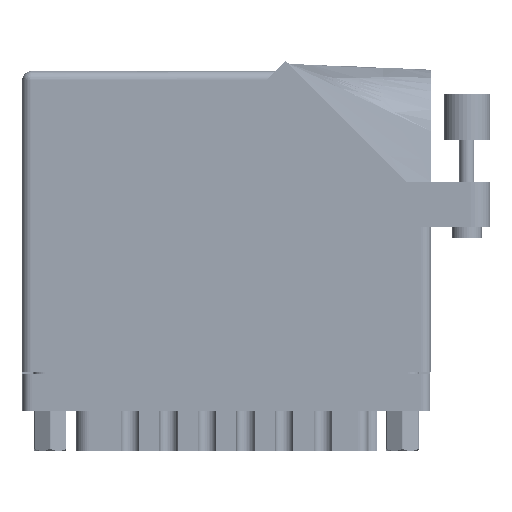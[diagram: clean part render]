
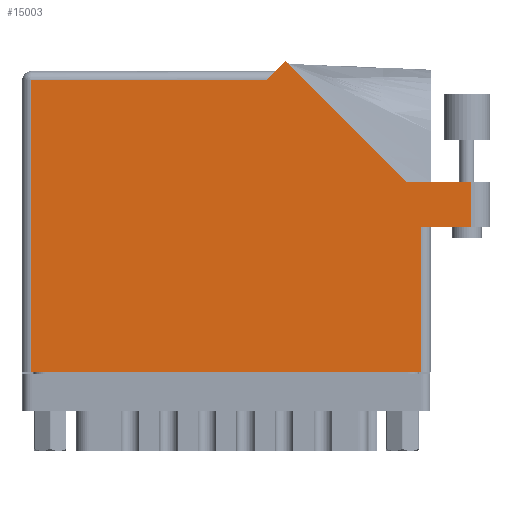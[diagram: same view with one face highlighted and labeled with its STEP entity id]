
A CAD part, front view. The second image highlights one B-rep face of the part: STEP entity #15003.
In plain terms, the highlighted face is planar.
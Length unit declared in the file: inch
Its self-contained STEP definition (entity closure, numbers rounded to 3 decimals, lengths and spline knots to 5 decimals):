
#31 = VECTOR ( 'NONE', #86775, 39.37008 ) ;
#2384 = ORIENTED_EDGE ( 'NONE', *, *, #24956, .T. ) ;
#2831 = ORIENTED_EDGE ( 'NONE', *, *, #23127, .T. ) ;
#3071 = VERTEX_POINT ( 'NONE', #104858 ) ;
#3099 = VECTOR ( 'NONE', #7529, 39.37008 ) ;
#4959 = CARTESIAN_POINT ( 'NONE',  ( 2.693, 0.98, 0. ) ) ;
#7529 = DIRECTION ( 'NONE',  ( 0., -1., 0. ) ) ;
#8479 = EDGE_CURVE ( 'NONE', #53730, #66438, #96730, .T. ) ;
#8989 = ORIENTED_EDGE ( 'NONE', *, *, #78465, .T. ) ;
#9529 = VERTEX_POINT ( 'NONE', #45288 ) ;
#11699 = DIRECTION ( 'NONE',  ( -1., 0., 0. ) ) ;
#15003 = ADVANCED_FACE ( 'NONE', ( #39832 ), #72555, .F. ) ;
#15287 = CARTESIAN_POINT ( 'NONE',  ( 3.03, 0.98, 0. ) ) ;
#18448 = ORIENTED_EDGE ( 'NONE', *, *, #77657, .T. ) ;
#19080 = AXIS2_PLACEMENT_3D ( 'NONE', #99212, #79554, #82600 ) ;
#19492 = EDGE_CURVE ( 'NONE', #73063, #45095, #75893, .T. ) ;
#23109 = CARTESIAN_POINT ( 'NONE',  ( 0.062, 0., 0. ) ) ;
#23127 = EDGE_CURVE ( 'NONE', #98525, #55032, #56002, .T. ) ;
#23287 = EDGE_LOOP ( 'NONE', ( #50645, #2831, #2384, #96172, #70123, #18448, #8989, #60711, #58109 ) ) ;
#24956 = EDGE_CURVE ( 'NONE', #55032, #73063, #66088, .T. ) ;
#28691 = VECTOR ( 'NONE', #67126, 39.37008 ) ;
#31933 = EDGE_CURVE ( 'NONE', #45095, #74661, #101680, .T. ) ;
#32439 = CARTESIAN_POINT ( 'NONE',  ( 1.77571, 2.10071, 0. ) ) ;
#35107 = DIRECTION ( 'NONE',  ( -0.707, 0.707, 0. ) ) ;
#37134 = EDGE_CURVE ( 'NONE', #3071, #53730, #75063, .T. ) ;
#37437 = CARTESIAN_POINT ( 'NONE',  ( 0., 1.968, 0. ) ) ;
#39832 = FACE_OUTER_BOUND ( 'NONE', #23287, .T. ) ;
#41699 = CARTESIAN_POINT ( 'NONE',  ( 3.03, 1.287, 0. ) ) ;
#41832 = VECTOR ( 'NONE', #35107, 39.37008 ) ;
#45095 = VERTEX_POINT ( 'NONE', #32439 ) ;
#45288 = CARTESIAN_POINT ( 'NONE',  ( 0.062, 1.968, 0. ) ) ;
#47624 = VECTOR ( 'NONE', #97640, 39.37008 ) ;
#50645 = ORIENTED_EDGE ( 'NONE', *, *, #66693, .T. ) ;
#53121 = CARTESIAN_POINT ( 'NONE',  ( 2.693, 0.98, 0. ) ) ;
#53528 = LINE ( 'NONE', #101830, #31 ) ;
#53730 = VERTEX_POINT ( 'NONE', #94861 ) ;
#55032 = VERTEX_POINT ( 'NONE', #41699 ) ;
#56002 = LINE ( 'NONE', #103795, #76701 ) ;
#57508 = CARTESIAN_POINT ( 'NONE',  ( 3.155, 1.287, 0. ) ) ;
#57904 = CARTESIAN_POINT ( 'NONE',  ( 0., 0., 0. ) ) ;
#58109 = ORIENTED_EDGE ( 'NONE', *, *, #8479, .T. ) ;
#60711 = ORIENTED_EDGE ( 'NONE', *, *, #37134, .T. ) ;
#63517 = DIRECTION ( 'NONE',  ( 0., 1., 0. ) ) ;
#66088 = LINE ( 'NONE', #57508, #28691 ) ;
#66121 = DIRECTION ( 'NONE',  ( 0., 1., 0. ) ) ;
#66438 = VERTEX_POINT ( 'NONE', #53121 ) ;
#66693 = EDGE_CURVE ( 'NONE', #66438, #98525, #53528, .T. ) ;
#67126 = DIRECTION ( 'NONE',  ( -1., 0., 0. ) ) ;
#70123 = ORIENTED_EDGE ( 'NONE', *, *, #31933, .T. ) ;
#72555 = PLANE ( 'NONE',  #19080 ) ;
#73063 = VERTEX_POINT ( 'NONE', #93005 ) ;
#74661 = VERTEX_POINT ( 'NONE', #93494 ) ;
#75063 = LINE ( 'NONE', #57904, #47624 ) ;
#75893 = LINE ( 'NONE', #85526, #41832 ) ;
#76664 = LINE ( 'NONE', #37437, #97178 ) ;
#76701 = VECTOR ( 'NONE', #63517, 39.37008 ) ;
#77657 = EDGE_CURVE ( 'NONE', #74661, #9529, #76664, .T. ) ;
#78465 = EDGE_CURVE ( 'NONE', #9529, #3071, #88592, .T. ) ;
#79554 = DIRECTION ( 'NONE',  ( 0., 0., -1. ) ) ;
#81264 = VECTOR ( 'NONE', #93096, 39.37008 ) ;
#82600 = DIRECTION ( 'NONE',  ( -1., 0., 0. ) ) ;
#85526 = CARTESIAN_POINT ( 'NONE',  ( 2.58942, 1.287, 0. ) ) ;
#85580 = CARTESIAN_POINT ( 'NONE',  ( 1.705, 2.03, 0. ) ) ;
#85784 = VECTOR ( 'NONE', #66121, 39.37008 ) ;
#86775 = DIRECTION ( 'NONE',  ( 1., 0., 0. ) ) ;
#88592 = LINE ( 'NONE', #23109, #3099 ) ;
#93005 = CARTESIAN_POINT ( 'NONE',  ( 2.58942, 1.287, 0. ) ) ;
#93096 = DIRECTION ( 'NONE',  ( -0.707, -0.707, 0. ) ) ;
#93494 = CARTESIAN_POINT ( 'NONE',  ( 1.643, 1.968, 0. ) ) ;
#94861 = CARTESIAN_POINT ( 'NONE',  ( 2.693, 0., 0. ) ) ;
#96172 = ORIENTED_EDGE ( 'NONE', *, *, #19492, .T. ) ;
#96730 = LINE ( 'NONE', #4959, #85784 ) ;
#97178 = VECTOR ( 'NONE', #11699, 39.37008 ) ;
#97640 = DIRECTION ( 'NONE',  ( 1., 0., 0. ) ) ;
#98525 = VERTEX_POINT ( 'NONE', #15287 ) ;
#99212 = CARTESIAN_POINT ( 'NONE',  ( 0., 2.03, 0. ) ) ;
#101680 = LINE ( 'NONE', #85580, #81264 ) ;
#101830 = CARTESIAN_POINT ( 'NONE',  ( 2.755, 0.98, 0. ) ) ;
#103795 = CARTESIAN_POINT ( 'NONE',  ( 3.03, 1.287, 0. ) ) ;
#104858 = CARTESIAN_POINT ( 'NONE',  ( 0.062, 0., 0. ) ) ;
